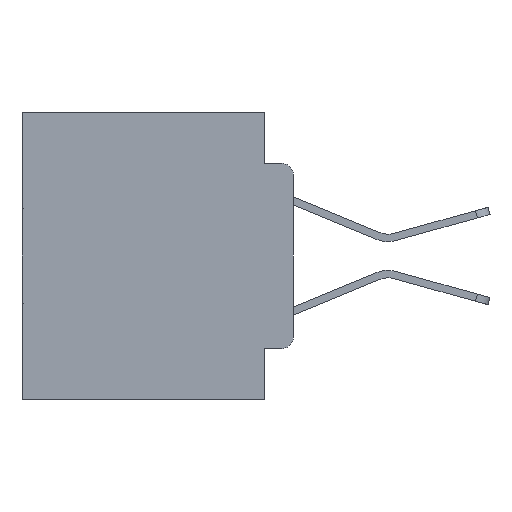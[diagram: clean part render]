
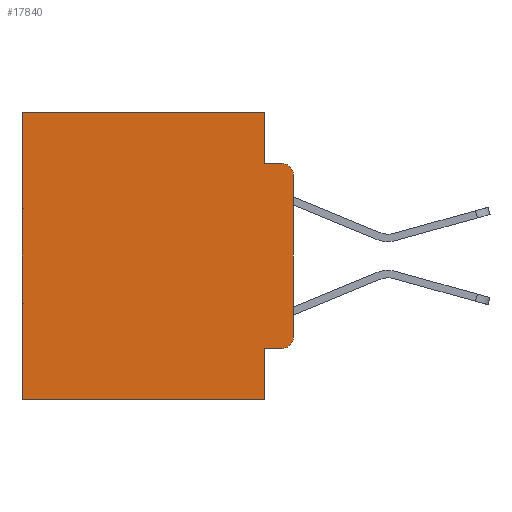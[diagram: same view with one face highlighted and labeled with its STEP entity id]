
A CAD part, left-side view. The second image highlights one B-rep face of the part: STEP entity #17840.
In plain terms, the highlighted planar face has unit normal (-1, 0, 0).
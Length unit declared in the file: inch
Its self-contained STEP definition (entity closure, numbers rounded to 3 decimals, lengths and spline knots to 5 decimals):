
#67 = DIRECTION ( 'NONE',  ( 0., 0., -1. ) ) ;
#1133 = VERTEX_POINT ( 'NONE', #22778 ) ;
#1334 = ORIENTED_EDGE ( 'NONE', *, *, #26344, .T. ) ;
#1917 = VECTOR ( 'NONE', #26257, 39.37008 ) ;
#2293 = EDGE_LOOP ( 'NONE', ( #14308, #5603, #2692, #29431, #1334, #16610, #23403, #14609, #10352, #18404 ) ) ;
#2692 = ORIENTED_EDGE ( 'NONE', *, *, #20900, .F. ) ;
#2774 = CARTESIAN_POINT ( 'NONE',  ( 0.298, 0., 0. ) ) ;
#3658 = DIRECTION ( 'NONE',  ( 0., 0., -1. ) ) ;
#3931 = CARTESIAN_POINT ( 'NONE',  ( 0.298, 0.051, -0.4115 ) ) ;
#4335 = CARTESIAN_POINT ( 'NONE',  ( 0.298, 0.02, -0.1085 ) ) ;
#4682 = DIRECTION ( 'NONE',  ( 0., 0., -1. ) ) ;
#4739 = VERTEX_POINT ( 'NONE', #23009 ) ;
#5279 = CIRCLE ( 'NONE', #12624, 0.02 ) ;
#5295 = DIRECTION ( 'NONE',  ( 1., 0., 0. ) ) ;
#5449 = VERTEX_POINT ( 'NONE', #20858 ) ;
#5603 = ORIENTED_EDGE ( 'NONE', *, *, #12772, .T. ) ;
#6646 = EDGE_CURVE ( 'NONE', #12596, #7048, #24151, .T. ) ;
#6841 = VECTOR ( 'NONE', #15603, 39.37008 ) ;
#7048 = VERTEX_POINT ( 'NONE', #18261 ) ;
#7055 = CARTESIAN_POINT ( 'NONE',  ( 0.298, 0.051, 0. ) ) ;
#7079 = CARTESIAN_POINT ( 'NONE',  ( 0.298, 0., 0. ) ) ;
#7608 = CARTESIAN_POINT ( 'NONE',  ( 0.298, 0., -0.5 ) ) ;
#7696 = PLANE ( 'NONE',  #10541 ) ;
#8081 = CARTESIAN_POINT ( 'NONE',  ( 0.298, 0., -0.3915 ) ) ;
#9136 = VECTOR ( 'NONE', #24543, 39.37008 ) ;
#9253 = DIRECTION ( 'NONE',  ( -1., 0., 0. ) ) ;
#9480 = VECTOR ( 'NONE', #22470, 39.37008 ) ;
#9672 = CARTESIAN_POINT ( 'NONE',  ( 0.298, 0.02, -0.4115 ) ) ;
#9831 = EDGE_CURVE ( 'NONE', #1133, #13899, #23928, .T. ) ;
#10246 = EDGE_CURVE ( 'NONE', #12596, #10638, #26932, .T. ) ;
#10352 = ORIENTED_EDGE ( 'NONE', *, *, #10246, .T. ) ;
#10541 = AXIS2_PLACEMENT_3D ( 'NONE', #2774, #5295, #26734 ) ;
#10638 = VERTEX_POINT ( 'NONE', #9672 ) ;
#11618 = VECTOR ( 'NONE', #4682, 39.37008 ) ;
#11793 = EDGE_CURVE ( 'NONE', #7048, #5449, #24529, .T. ) ;
#12447 = LINE ( 'NONE', #22672, #9480 ) ;
#12596 = VERTEX_POINT ( 'NONE', #3931 ) ;
#12624 = AXIS2_PLACEMENT_3D ( 'NONE', #24969, #12848, #3658 ) ;
#12772 = EDGE_CURVE ( 'NONE', #21349, #4739, #28310, .T. ) ;
#12848 = DIRECTION ( 'NONE',  ( -1., 0., 0. ) ) ;
#13199 = EDGE_CURVE ( 'NONE', #17851, #5449, #12447, .T. ) ;
#13322 = CARTESIAN_POINT ( 'NONE',  ( 0.298, 0.051, -0.4115 ) ) ;
#13380 = VECTOR ( 'NONE', #67, 39.37008 ) ;
#13721 = EDGE_CURVE ( 'NONE', #10638, #24308, #5279, .T. ) ;
#13899 = VERTEX_POINT ( 'NONE', #27827 ) ;
#14308 = ORIENTED_EDGE ( 'NONE', *, *, #27204, .F. ) ;
#14406 = CARTESIAN_POINT ( 'NONE',  ( 0.298, 0., 0. ) ) ;
#14609 = ORIENTED_EDGE ( 'NONE', *, *, #6646, .F. ) ;
#15603 = DIRECTION ( 'NONE',  ( 0., 0., -1. ) ) ;
#16226 = DIRECTION ( 'NONE',  ( 0., 1., 0. ) ) ;
#16610 = ORIENTED_EDGE ( 'NONE', *, *, #13199, .T. ) ;
#17840 = ADVANCED_FACE ( 'NONE', ( #21284 ), #7696, .F. ) ;
#17851 = VERTEX_POINT ( 'NONE', #19688 ) ;
#18261 = CARTESIAN_POINT ( 'NONE',  ( 0.298, 0.051, -0.5 ) ) ;
#18393 = DIRECTION ( 'NONE',  ( 0., 0., -1. ) ) ;
#18404 = ORIENTED_EDGE ( 'NONE', *, *, #13721, .T. ) ;
#18992 = CARTESIAN_POINT ( 'NONE',  ( 0.298, 0.051, -0.0885 ) ) ;
#19688 = CARTESIAN_POINT ( 'NONE',  ( 0.298, 0.473, 0. ) ) ;
#20536 = VECTOR ( 'NONE', #20722, 39.37008 ) ;
#20722 = DIRECTION ( 'NONE',  ( 0., -1., 0. ) ) ;
#20858 = CARTESIAN_POINT ( 'NONE',  ( 0.298, 0.473, -0.5 ) ) ;
#20900 = EDGE_CURVE ( 'NONE', #13899, #4739, #28605, .T. ) ;
#21284 = FACE_OUTER_BOUND ( 'NONE', #2293, .T. ) ;
#21349 = VERTEX_POINT ( 'NONE', #27831 ) ;
#22470 = DIRECTION ( 'NONE',  ( 0., 0., -1. ) ) ;
#22672 = CARTESIAN_POINT ( 'NONE',  ( 0.298, 0.473, 0. ) ) ;
#22778 = CARTESIAN_POINT ( 'NONE',  ( 0.298, 0.051, 0. ) ) ;
#23009 = CARTESIAN_POINT ( 'NONE',  ( 0.298, 0.02, -0.0885 ) ) ;
#23403 = ORIENTED_EDGE ( 'NONE', *, *, #11793, .F. ) ;
#23928 = LINE ( 'NONE', #7055, #13380 ) ;
#24151 = LINE ( 'NONE', #25082, #6841 ) ;
#24308 = VERTEX_POINT ( 'NONE', #8081 ) ;
#24529 = LINE ( 'NONE', #7608, #9136 ) ;
#24543 = DIRECTION ( 'NONE',  ( 0., 1., 0. ) ) ;
#24826 = LINE ( 'NONE', #7079, #27119 ) ;
#24969 = CARTESIAN_POINT ( 'NONE',  ( 0.298, 0.02, -0.3915 ) ) ;
#25082 = CARTESIAN_POINT ( 'NONE',  ( 0.298, 0.051, 0. ) ) ;
#26257 = DIRECTION ( 'NONE',  ( 0., -1., 0. ) ) ;
#26338 = AXIS2_PLACEMENT_3D ( 'NONE', #4335, #9253, #18393 ) ;
#26344 = EDGE_CURVE ( 'NONE', #1133, #17851, #24826, .T. ) ;
#26734 = DIRECTION ( 'NONE',  ( 0., 0., -1. ) ) ;
#26932 = LINE ( 'NONE', #13322, #20536 ) ;
#27119 = VECTOR ( 'NONE', #16226, 39.37008 ) ;
#27204 = EDGE_CURVE ( 'NONE', #21349, #24308, #30780, .T. ) ;
#27827 = CARTESIAN_POINT ( 'NONE',  ( 0.298, 0.051, -0.0885 ) ) ;
#27831 = CARTESIAN_POINT ( 'NONE',  ( 0.298, 0., -0.1085 ) ) ;
#28310 = CIRCLE ( 'NONE', #26338, 0.02 ) ;
#28605 = LINE ( 'NONE', #18992, #1917 ) ;
#29431 = ORIENTED_EDGE ( 'NONE', *, *, #9831, .F. ) ;
#30780 = LINE ( 'NONE', #14406, #11618 ) ;
